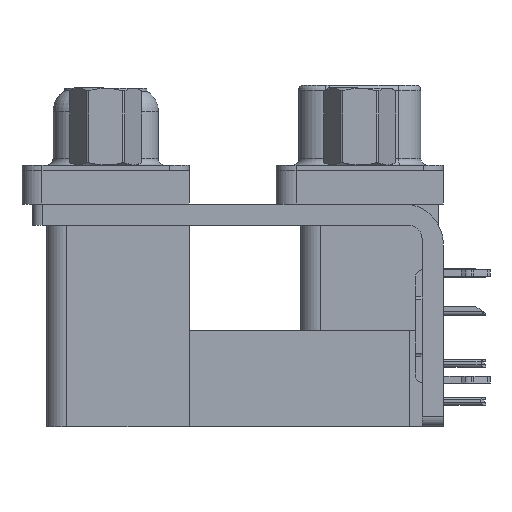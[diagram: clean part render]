
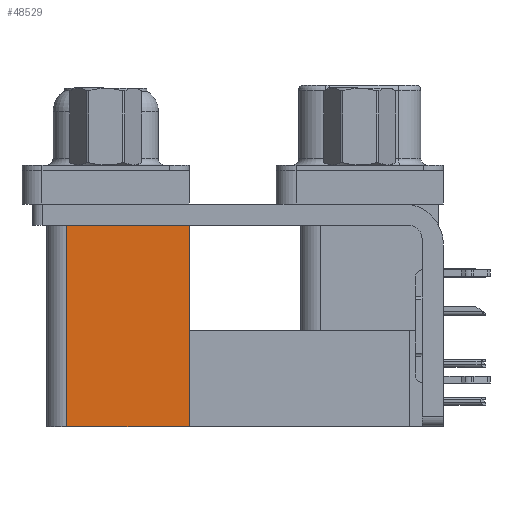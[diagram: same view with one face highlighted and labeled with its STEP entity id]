
A CAD part, left-side view. The second image highlights one B-rep face of the part: STEP entity #48529.
In plain terms, the highlighted planar face has unit normal (-1, 0, 0).
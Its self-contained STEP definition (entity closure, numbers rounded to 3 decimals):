
#1500 = ORIENTED_EDGE ( 'NONE', *, *, #45671, .T. ) ;
#3022 = CARTESIAN_POINT ( 'NONE',  ( 3.765, 21.975, -2.5 ) ) ;
#3072 = VERTEX_POINT ( 'NONE', #28438 ) ;
#4031 = DIRECTION ( 'NONE',  ( 1., 0., 0. ) ) ;
#4550 = VERTEX_POINT ( 'NONE', #45397 ) ;
#8193 = FACE_OUTER_BOUND ( 'NONE', #32640, .T. ) ;
#9768 = VERTEX_POINT ( 'NONE', #18737 ) ;
#9847 = LINE ( 'NONE', #33312, #37026 ) ;
#13010 = AXIS2_PLACEMENT_3D ( 'NONE', #23304, #4031, #39961 ) ;
#15219 = VECTOR ( 'NONE', #48133, 1000. ) ;
#15279 = EDGE_CURVE ( 'NONE', #3072, #17152, #29144, .T. ) ;
#15362 = ORIENTED_EDGE ( 'NONE', *, *, #40140, .F. ) ;
#16362 = CARTESIAN_POINT ( 'NONE',  ( 3.765, 12.775, -2.5 ) ) ;
#17128 = DIRECTION ( 'NONE',  ( 0., 1., 0. ) ) ;
#17152 = VERTEX_POINT ( 'NONE', #3022 ) ;
#18502 = LINE ( 'NONE', #30754, #31290 ) ;
#18737 = CARTESIAN_POINT ( 'NONE',  ( 3.765, 21.975, -19.2 ) ) ;
#19796 = ORIENTED_EDGE ( 'NONE', *, *, #15279, .T. ) ;
#23304 = CARTESIAN_POINT ( 'NONE',  ( 3.765, 12.775, -19.2 ) ) ;
#23564 = PLANE ( 'NONE',  #13010 ) ;
#26257 = ORIENTED_EDGE ( 'NONE', *, *, #48304, .F. ) ;
#26353 = DIRECTION ( 'NONE',  ( 0., 0., 1. ) ) ;
#26975 = LINE ( 'NONE', #42601, #47062 ) ;
#28438 = CARTESIAN_POINT ( 'NONE',  ( 3.765, 12.775, -2.5 ) ) ;
#29144 = LINE ( 'NONE', #16362, #15219 ) ;
#30754 = CARTESIAN_POINT ( 'NONE',  ( 3.765, 12.775, -19.2 ) ) ;
#31290 = VECTOR ( 'NONE', #26353, 1000. ) ;
#32640 = EDGE_LOOP ( 'NONE', ( #19796, #26257, #15362, #1500 ) ) ;
#33312 = CARTESIAN_POINT ( 'NONE',  ( 3.765, 12.775, -19.2 ) ) ;
#37026 = VECTOR ( 'NONE', #17128, 1000. ) ;
#39961 = DIRECTION ( 'NONE',  ( 0., 1., 0. ) ) ;
#40140 = EDGE_CURVE ( 'NONE', #4550, #9768, #9847, .T. ) ;
#42601 = CARTESIAN_POINT ( 'NONE',  ( 3.765, 21.975, -19.2 ) ) ;
#42857 = DIRECTION ( 'NONE',  ( 0., 0., 1. ) ) ;
#45397 = CARTESIAN_POINT ( 'NONE',  ( 3.765, 12.775, -19.2 ) ) ;
#45671 = EDGE_CURVE ( 'NONE', #4550, #3072, #18502, .T. ) ;
#47062 = VECTOR ( 'NONE', #42857, 1000. ) ;
#48133 = DIRECTION ( 'NONE',  ( 0., 1., 0. ) ) ;
#48304 = EDGE_CURVE ( 'NONE', #9768, #17152, #26975, .T. ) ;
#48529 = ADVANCED_FACE ( 'NONE', ( #8193 ), #23564, .F. ) ;
